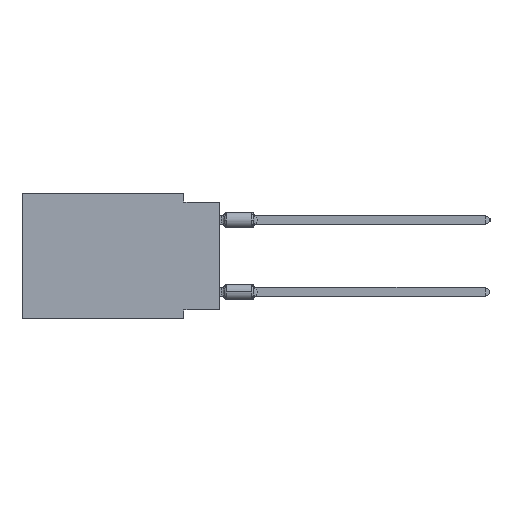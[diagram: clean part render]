
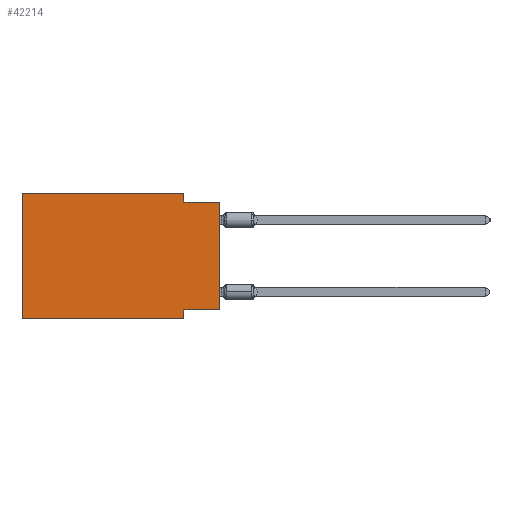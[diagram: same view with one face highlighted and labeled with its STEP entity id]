
A CAD part, left-side view. The second image highlights one B-rep face of the part: STEP entity #42214.
In plain terms, the highlighted planar face has unit normal (-1, 0, 0).
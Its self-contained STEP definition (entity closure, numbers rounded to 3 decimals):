
#675 = VERTEX_POINT ( 'NONE', #11080 ) ;
#863 = EDGE_CURVE ( 'NONE', #24950, #43164, #29919, .T. ) ;
#1106 = VECTOR ( 'NONE', #3162, 1000. ) ;
#1501 = VECTOR ( 'NONE', #12811, 1000. ) ;
#1706 = DIRECTION ( 'NONE',  ( 0., 0., -1. ) ) ;
#2933 = CARTESIAN_POINT ( 'NONE',  ( 0., 13.97, 0. ) ) ;
#3162 = DIRECTION ( 'NONE',  ( 0., -1., 0. ) ) ;
#3614 = VERTEX_POINT ( 'NONE', #37403 ) ;
#5088 = ORIENTED_EDGE ( 'NONE', *, *, #863, .T. ) ;
#6394 = EDGE_CURVE ( 'NONE', #25564, #3614, #13419, .T. ) ;
#6759 = CARTESIAN_POINT ( 'NONE',  ( 0., 0., 0. ) ) ;
#6949 = VERTEX_POINT ( 'NONE', #39615 ) ;
#6996 = CARTESIAN_POINT ( 'NONE',  ( 0., 13.97, 0. ) ) ;
#7021 = VECTOR ( 'NONE', #34418, 1000. ) ;
#7556 = AXIS2_PLACEMENT_3D ( 'NONE', #43347, #19530, #33250 ) ;
#7696 = CARTESIAN_POINT ( 'NONE',  ( 0., 13.97, -8.89 ) ) ;
#8742 = VECTOR ( 'NONE', #17313, 1000. ) ;
#9703 = VECTOR ( 'NONE', #22409, 1000. ) ;
#11017 = VECTOR ( 'NONE', #37464, 1000. ) ;
#11080 = CARTESIAN_POINT ( 'NONE',  ( 0., 2.54, -8.255 ) ) ;
#11340 = ORIENTED_EDGE ( 'NONE', *, *, #32090, .F. ) ;
#11494 = ORIENTED_EDGE ( 'NONE', *, *, #34061, .F. ) ;
#12811 = DIRECTION ( 'NONE',  ( 0., 1., 0. ) ) ;
#13419 = LINE ( 'NONE', #27141, #11017 ) ;
#13934 = VERTEX_POINT ( 'NONE', #2933 ) ;
#15449 = LINE ( 'NONE', #36557, #9703 ) ;
#15532 = CARTESIAN_POINT ( 'NONE',  ( 0., 0., -8.255 ) ) ;
#16204 = LINE ( 'NONE', #15532, #1501 ) ;
#17313 = DIRECTION ( 'NONE',  ( 0., 0., 1. ) ) ;
#17942 = CARTESIAN_POINT ( 'NONE',  ( 0., 0., -0.635 ) ) ;
#18111 = ORIENTED_EDGE ( 'NONE', *, *, #20703, .F. ) ;
#18448 = EDGE_CURVE ( 'NONE', #13934, #25564, #37787, .T. ) ;
#19226 = ORIENTED_EDGE ( 'NONE', *, *, #42615, .F. ) ;
#19530 = DIRECTION ( 'NONE',  ( 1., 0., 0. ) ) ;
#20490 = CARTESIAN_POINT ( 'NONE',  ( 0., 2.54, -8.89 ) ) ;
#20703 = EDGE_CURVE ( 'NONE', #24950, #13934, #22266, .T. ) ;
#21592 = VECTOR ( 'NONE', #1706, 1000. ) ;
#22266 = LINE ( 'NONE', #36639, #32222 ) ;
#22371 = LINE ( 'NONE', #32483, #21592 ) ;
#22409 = DIRECTION ( 'NONE',  ( 0., -1., 0. ) ) ;
#24118 = EDGE_LOOP ( 'NONE', ( #42388, #19226, #41940, #41625, #18111, #5088, #11340, #11494 ) ) ;
#24950 = VERTEX_POINT ( 'NONE', #7696 ) ;
#25564 = VERTEX_POINT ( 'NONE', #25762 ) ;
#25762 = CARTESIAN_POINT ( 'NONE',  ( 0., 2.54, 0. ) ) ;
#27141 = CARTESIAN_POINT ( 'NONE',  ( 0., 2.54, 0. ) ) ;
#29663 = FACE_OUTER_BOUND ( 'NONE', #24118, .T. ) ;
#29919 = LINE ( 'NONE', #40220, #1106 ) ;
#31467 = VERTEX_POINT ( 'NONE', #17942 ) ;
#32090 = EDGE_CURVE ( 'NONE', #675, #43164, #22371, .T. ) ;
#32222 = VECTOR ( 'NONE', #35981, 1000. ) ;
#32483 = CARTESIAN_POINT ( 'NONE',  ( 0., 2.54, -8.89 ) ) ;
#33250 = DIRECTION ( 'NONE',  ( 0., 0., -1. ) ) ;
#34061 = EDGE_CURVE ( 'NONE', #6949, #675, #16204, .T. ) ;
#34418 = DIRECTION ( 'NONE',  ( 0., -1., 0. ) ) ;
#35367 = EDGE_CURVE ( 'NONE', #6949, #31467, #40688, .T. ) ;
#35981 = DIRECTION ( 'NONE',  ( 0., 0., 1. ) ) ;
#36557 = CARTESIAN_POINT ( 'NONE',  ( 0., 0., -0.635 ) ) ;
#36611 = PLANE ( 'NONE',  #7556 ) ;
#36639 = CARTESIAN_POINT ( 'NONE',  ( 0., 13.97, 0. ) ) ;
#37403 = CARTESIAN_POINT ( 'NONE',  ( 0., 2.54, -0.635 ) ) ;
#37464 = DIRECTION ( 'NONE',  ( 0., 0., -1. ) ) ;
#37787 = LINE ( 'NONE', #6996, #7021 ) ;
#39615 = CARTESIAN_POINT ( 'NONE',  ( 0., 0., -8.255 ) ) ;
#40220 = CARTESIAN_POINT ( 'NONE',  ( 0., 13.97, -8.89 ) ) ;
#40688 = LINE ( 'NONE', #6759, #8742 ) ;
#41625 = ORIENTED_EDGE ( 'NONE', *, *, #18448, .F. ) ;
#41940 = ORIENTED_EDGE ( 'NONE', *, *, #6394, .F. ) ;
#42214 = ADVANCED_FACE ( 'NONE', ( #29663 ), #36611, .F. ) ;
#42388 = ORIENTED_EDGE ( 'NONE', *, *, #35367, .T. ) ;
#42615 = EDGE_CURVE ( 'NONE', #3614, #31467, #15449, .T. ) ;
#43164 = VERTEX_POINT ( 'NONE', #20490 ) ;
#43347 = CARTESIAN_POINT ( 'NONE',  ( 0., 13.97, 0. ) ) ;
